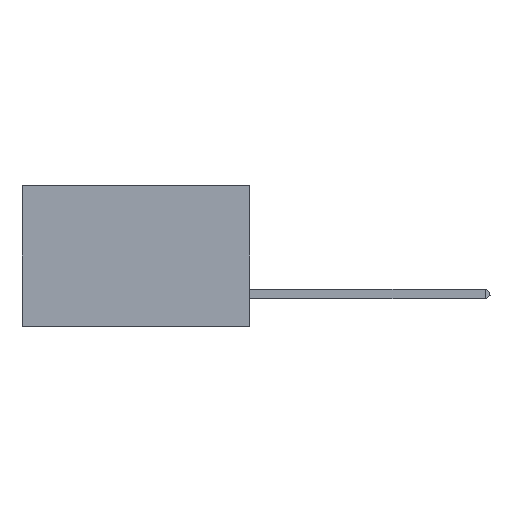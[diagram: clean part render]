
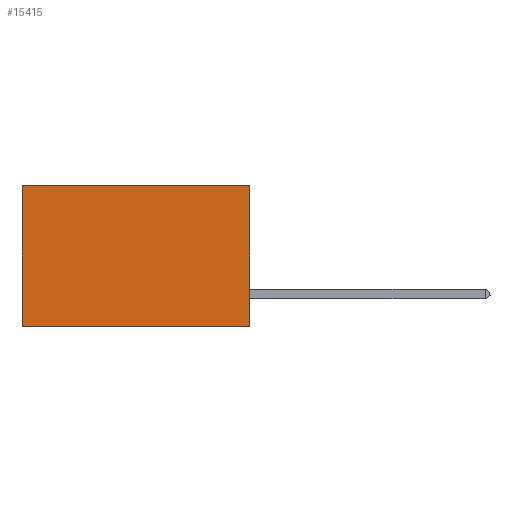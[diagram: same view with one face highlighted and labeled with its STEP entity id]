
A CAD part, left-side view. The second image highlights one B-rep face of the part: STEP entity #15415.
In plain terms, the highlighted planar face has unit normal (-1, 0, 0).
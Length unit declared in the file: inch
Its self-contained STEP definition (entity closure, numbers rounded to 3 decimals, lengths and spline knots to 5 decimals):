
#485 = CARTESIAN_POINT ( 'NONE',  ( 0.2875, 0., 0. ) ) ;
#697 = PLANE ( 'NONE',  #16205 ) ;
#2065 = VERTEX_POINT ( 'NONE', #4228 ) ;
#2508 = DIRECTION ( 'NONE',  ( 0., 0., -1. ) ) ;
#2736 = LINE ( 'NONE', #7384, #23030 ) ;
#4228 = CARTESIAN_POINT ( 'NONE',  ( 0.2875, 0., -0.37 ) ) ;
#4283 = VERTEX_POINT ( 'NONE', #485 ) ;
#4782 = EDGE_CURVE ( 'NONE', #4283, #2065, #9182, .T. ) ;
#5251 = ORIENTED_EDGE ( 'NONE', *, *, #20110, .F. ) ;
#6048 = VECTOR ( 'NONE', #21737, 39.37008 ) ;
#6279 = EDGE_CURVE ( 'NONE', #4283, #20443, #17569, .T. ) ;
#7316 = CARTESIAN_POINT ( 'NONE',  ( 0.2875, 0.6, -0.37 ) ) ;
#7384 = CARTESIAN_POINT ( 'NONE',  ( 0.2875, 0.6, 0. ) ) ;
#7565 = ORIENTED_EDGE ( 'NONE', *, *, #4782, .F. ) ;
#9120 = VECTOR ( 'NONE', #10419, 39.37008 ) ;
#9182 = LINE ( 'NONE', #12483, #6048 ) ;
#9260 = ORIENTED_EDGE ( 'NONE', *, *, #21229, .T. ) ;
#10419 = DIRECTION ( 'NONE',  ( 0., 1., 0. ) ) ;
#11733 = EDGE_LOOP ( 'NONE', ( #9260, #5251, #7565, #17105 ) ) ;
#12109 = DIRECTION ( 'NONE',  ( 0., 1., 0. ) ) ;
#12300 = DIRECTION ( 'NONE',  ( 0., 0., -1. ) ) ;
#12483 = CARTESIAN_POINT ( 'NONE',  ( 0.2875, 0., 0. ) ) ;
#14451 = CARTESIAN_POINT ( 'NONE',  ( 0.2875, 0.6, 0. ) ) ;
#14564 = VECTOR ( 'NONE', #12109, 39.37008 ) ;
#15415 = ADVANCED_FACE ( 'NONE', ( #19625 ), #697, .F. ) ;
#15602 = CARTESIAN_POINT ( 'NONE',  ( 0.2875, 0., -0.37 ) ) ;
#16205 = AXIS2_PLACEMENT_3D ( 'NONE', #22188, #16749, #2508 ) ;
#16749 = DIRECTION ( 'NONE',  ( 1., 0., 0. ) ) ;
#16819 = LINE ( 'NONE', #15602, #14564 ) ;
#17105 = ORIENTED_EDGE ( 'NONE', *, *, #6279, .T. ) ;
#17213 = VERTEX_POINT ( 'NONE', #7316 ) ;
#17569 = LINE ( 'NONE', #22520, #9120 ) ;
#19625 = FACE_OUTER_BOUND ( 'NONE', #11733, .T. ) ;
#20110 = EDGE_CURVE ( 'NONE', #2065, #17213, #16819, .T. ) ;
#20443 = VERTEX_POINT ( 'NONE', #14451 ) ;
#21229 = EDGE_CURVE ( 'NONE', #20443, #17213, #2736, .T. ) ;
#21737 = DIRECTION ( 'NONE',  ( 0., 0., -1. ) ) ;
#22188 = CARTESIAN_POINT ( 'NONE',  ( 0.2875, 0., 0. ) ) ;
#22520 = CARTESIAN_POINT ( 'NONE',  ( 0.2875, 0., 0. ) ) ;
#23030 = VECTOR ( 'NONE', #12300, 39.37008 ) ;
